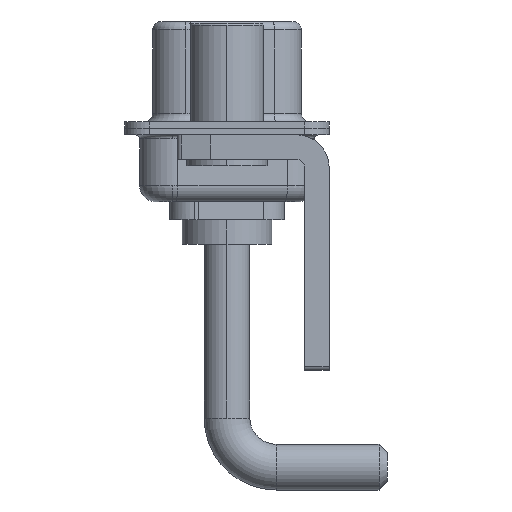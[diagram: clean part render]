
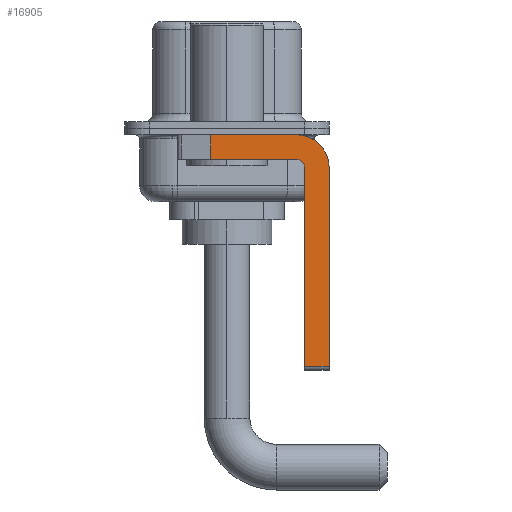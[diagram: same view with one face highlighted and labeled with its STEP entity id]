
A CAD part, left-side view. The second image highlights one B-rep face of the part: STEP entity #16905.
In plain terms, the highlighted planar face has unit normal (-1, 0, 0).
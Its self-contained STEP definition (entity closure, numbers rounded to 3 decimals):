
#63 = VERTEX_POINT ( 'NONE', #15540 ) ;
#1144 = AXIS2_PLACEMENT_3D ( 'NONE', #5005, #10650, #3432 ) ;
#1940 = CARTESIAN_POINT ( 'NONE',  ( -2.9, -4.25, -1.9 ) ) ;
#2020 = FACE_OUTER_BOUND ( 'NONE', #5359, .T. ) ;
#2202 = LINE ( 'NONE', #3605, #8105 ) ;
#2528 = VERTEX_POINT ( 'NONE', #2677 ) ;
#2677 = CARTESIAN_POINT ( 'NONE',  ( -2.9, -4.75, -14.55 ) ) ;
#2721 = CARTESIAN_POINT ( 'NONE',  ( -2.9, 3., -0.4 ) ) ;
#2851 = ORIENTED_EDGE ( 'NONE', *, *, #12805, .F. ) ;
#2957 = LINE ( 'NONE', #14451, #7953 ) ;
#3304 = EDGE_CURVE ( 'NONE', #63, #14104, #10495, .T. ) ;
#3432 = DIRECTION ( 'NONE',  ( 0., 0., -1. ) ) ;
#3605 = CARTESIAN_POINT ( 'NONE',  ( -2.9, -4.25, -14.55 ) ) ;
#3740 = EDGE_CURVE ( 'NONE', #2528, #9705, #2202, .T. ) ;
#3904 = DIRECTION ( 'NONE',  ( 0., 0., -1. ) ) ;
#4279 = DIRECTION ( 'NONE',  ( 0., 1., 0. ) ) ;
#4513 = EDGE_CURVE ( 'NONE', #16221, #63, #15632, .T. ) ;
#5005 = CARTESIAN_POINT ( 'NONE',  ( -2.9, -4.25, -2.4 ) ) ;
#5205 = DIRECTION ( 'NONE',  ( 1., 0., 0. ) ) ;
#5359 = EDGE_LOOP ( 'NONE', ( #8874, #7229, #16142, #2851, #5511, #18327, #10963, #13072 ) ) ;
#5511 = ORIENTED_EDGE ( 'NONE', *, *, #12044, .F. ) ;
#5516 = LINE ( 'NONE', #15989, #10056 ) ;
#6242 = LINE ( 'NONE', #14072, #8947 ) ;
#6400 = CARTESIAN_POINT ( 'NONE',  ( -2.9, -6.25, -2.4 ) ) ;
#7229 = ORIENTED_EDGE ( 'NONE', *, *, #8968, .T. ) ;
#7316 = VERTEX_POINT ( 'NONE', #1940 ) ;
#7553 = DIRECTION ( 'NONE',  ( 0., 0., -1. ) ) ;
#7870 = CARTESIAN_POINT ( 'NONE',  ( -2.9, -4.25, -2.4 ) ) ;
#7953 = VECTOR ( 'NONE', #7553, 1000. ) ;
#7963 = CARTESIAN_POINT ( 'NONE',  ( -2.9, -4.75, -2.4 ) ) ;
#8105 = VECTOR ( 'NONE', #11006, 1000. ) ;
#8205 = DIRECTION ( 'NONE',  ( 0., 0., 1. ) ) ;
#8314 = VECTOR ( 'NONE', #4279, 1000. ) ;
#8435 = DIRECTION ( 'NONE',  ( 0., -1., 0. ) ) ;
#8874 = ORIENTED_EDGE ( 'NONE', *, *, #4513, .F. ) ;
#8947 = VECTOR ( 'NONE', #8205, 1000. ) ;
#8968 = EDGE_CURVE ( 'NONE', #16221, #12622, #2957, .T. ) ;
#9467 = CIRCLE ( 'NONE', #16404, 0.5 ) ;
#9705 = VERTEX_POINT ( 'NONE', #10978 ) ;
#9898 = EDGE_CURVE ( 'NONE', #14104, #9705, #5516, .T. ) ;
#10056 = VECTOR ( 'NONE', #17675, 1000. ) ;
#10495 = CIRCLE ( 'NONE', #15343, 2. ) ;
#10520 = VECTOR ( 'NONE', #8435, 1000. ) ;
#10592 = DIRECTION ( 'NONE',  ( -1., 0., 0. ) ) ;
#10650 = DIRECTION ( 'NONE',  ( 1., 0., 0. ) ) ;
#10963 = ORIENTED_EDGE ( 'NONE', *, *, #9898, .F. ) ;
#10978 = CARTESIAN_POINT ( 'NONE',  ( -2.9, -6.25, -14.55 ) ) ;
#11006 = DIRECTION ( 'NONE',  ( 0., -1., 0. ) ) ;
#11326 = LINE ( 'NONE', #17006, #8314 ) ;
#11644 = EDGE_CURVE ( 'NONE', #7316, #12622, #11326, .T. ) ;
#12044 = EDGE_CURVE ( 'NONE', #2528, #12820, #6242, .T. ) ;
#12622 = VERTEX_POINT ( 'NONE', #14144 ) ;
#12805 = EDGE_CURVE ( 'NONE', #12820, #7316, #9467, .T. ) ;
#12820 = VERTEX_POINT ( 'NONE', #7963 ) ;
#13072 = ORIENTED_EDGE ( 'NONE', *, *, #3304, .F. ) ;
#13536 = DIRECTION ( 'NONE',  ( 0., 0., 1. ) ) ;
#14072 = CARTESIAN_POINT ( 'NONE',  ( -2.9, -4.75, -14.8 ) ) ;
#14104 = VERTEX_POINT ( 'NONE', #6400 ) ;
#14144 = CARTESIAN_POINT ( 'NONE',  ( -2.9, 0.978, -1.9 ) ) ;
#14451 = CARTESIAN_POINT ( 'NONE',  ( -2.9, 0.978, -1.9 ) ) ;
#15207 = PLANE ( 'NONE',  #1144 ) ;
#15343 = AXIS2_PLACEMENT_3D ( 'NONE', #18407, #5205, #3904 ) ;
#15540 = CARTESIAN_POINT ( 'NONE',  ( -2.9, -4.25, -0.4 ) ) ;
#15632 = LINE ( 'NONE', #2721, #10520 ) ;
#15989 = CARTESIAN_POINT ( 'NONE',  ( -2.9, -6.25, -2.4 ) ) ;
#16142 = ORIENTED_EDGE ( 'NONE', *, *, #11644, .F. ) ;
#16221 = VERTEX_POINT ( 'NONE', #17499 ) ;
#16404 = AXIS2_PLACEMENT_3D ( 'NONE', #7870, #10592, #13536 ) ;
#16905 = ADVANCED_FACE ( 'NONE', ( #2020 ), #15207, .F. ) ;
#17006 = CARTESIAN_POINT ( 'NONE',  ( -2.9, -4.25, -1.9 ) ) ;
#17499 = CARTESIAN_POINT ( 'NONE',  ( -2.9, 0.978, -0.4 ) ) ;
#17675 = DIRECTION ( 'NONE',  ( 0., 0., -1. ) ) ;
#18327 = ORIENTED_EDGE ( 'NONE', *, *, #3740, .T. ) ;
#18407 = CARTESIAN_POINT ( 'NONE',  ( -2.9, -4.25, -2.4 ) ) ;
